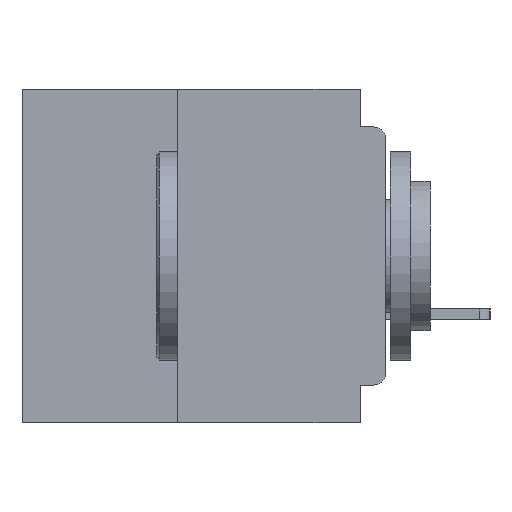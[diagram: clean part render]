
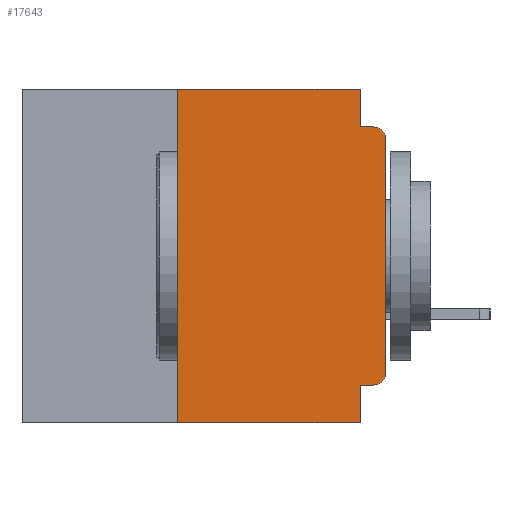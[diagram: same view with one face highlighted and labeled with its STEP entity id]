
A CAD part, left-side view. The second image highlights one B-rep face of the part: STEP entity #17643.
In plain terms, the highlighted planar face has unit normal (-1, 0, 0).
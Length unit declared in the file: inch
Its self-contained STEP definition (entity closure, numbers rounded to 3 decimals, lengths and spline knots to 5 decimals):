
#552 = DIRECTION ( 'NONE',  ( -1., 0., 0. ) ) ;
#1470 = LINE ( 'NONE', #4682, #11370 ) ;
#1479 = CARTESIAN_POINT ( 'NONE',  ( 0., 0.031, -0.4 ) ) ;
#1695 = DIRECTION ( 'NONE',  ( 0., 1., 0. ) ) ;
#1848 = VERTEX_POINT ( 'NONE', #18708 ) ;
#2295 = EDGE_CURVE ( 'NONE', #50090, #1848, #46483, .T. ) ;
#2937 = EDGE_CURVE ( 'NONE', #40375, #10852, #7028, .T. ) ;
#3346 = EDGE_CURVE ( 'NONE', #35002, #20147, #49579, .T. ) ;
#4307 = CARTESIAN_POINT ( 'NONE',  ( 0., 0., 0. ) ) ;
#4682 = CARTESIAN_POINT ( 'NONE',  ( 0., 0.031, 0. ) ) ;
#5439 = ORIENTED_EDGE ( 'NONE', *, *, #36839, .F. ) ;
#5777 = EDGE_CURVE ( 'NONE', #19562, #10852, #32001, .T. ) ;
#6863 = VERTEX_POINT ( 'NONE', #14213 ) ;
#7028 = LINE ( 'NONE', #52720, #16855 ) ;
#8505 = AXIS2_PLACEMENT_3D ( 'NONE', #49278, #53401, #28802 ) ;
#8623 = EDGE_CURVE ( 'NONE', #19562, #12308, #39413, .T. ) ;
#8981 = CIRCLE ( 'NONE', #23142, 0.015 ) ;
#8997 = ORIENTED_EDGE ( 'NONE', *, *, #5777, .T. ) ;
#9001 = EDGE_CURVE ( 'NONE', #17602, #1848, #8981, .T. ) ;
#10029 = VECTOR ( 'NONE', #27880, 39.37008 ) ;
#10455 = ORIENTED_EDGE ( 'NONE', *, *, #3346, .T. ) ;
#10621 = LINE ( 'NONE', #43025, #42249 ) ;
#10852 = VERTEX_POINT ( 'NONE', #1479 ) ;
#11066 = ORIENTED_EDGE ( 'NONE', *, *, #38443, .T. ) ;
#11228 = CARTESIAN_POINT ( 'NONE',  ( 0., 0.437, -0.4 ) ) ;
#11370 = VECTOR ( 'NONE', #25450, 39.37008 ) ;
#12308 = VERTEX_POINT ( 'NONE', #48574 ) ;
#12847 = CARTESIAN_POINT ( 'NONE',  ( 0., 0.015, -0.355 ) ) ;
#14213 = CARTESIAN_POINT ( 'NONE',  ( 0., 0.031, 0. ) ) ;
#14452 = CARTESIAN_POINT ( 'NONE',  ( 0., 0.25, -0.4 ) ) ;
#14571 = ORIENTED_EDGE ( 'NONE', *, *, #9001, .T. ) ;
#15018 = AXIS2_PLACEMENT_3D ( 'NONE', #42183, #42110, #41984 ) ;
#16855 = VECTOR ( 'NONE', #52776, 39.37008 ) ;
#17497 = EDGE_LOOP ( 'NONE', ( #11066, #14571, #36678, #48957, #5439, #48755, #8997, #39655, #50337, #10455 ) ) ;
#17602 = VERTEX_POINT ( 'NONE', #32575 ) ;
#17643 = ADVANCED_FACE ( 'NONE', ( #43228 ), #20543, .F. ) ;
#18305 = LINE ( 'NONE', #50562, #40161 ) ;
#18708 = CARTESIAN_POINT ( 'NONE',  ( 0., 0.015, -0.045 ) ) ;
#18836 = VECTOR ( 'NONE', #48781, 39.37008 ) ;
#19562 = VERTEX_POINT ( 'NONE', #28008 ) ;
#19796 = EDGE_CURVE ( 'NONE', #6863, #50090, #1470, .T. ) ;
#20147 = VERTEX_POINT ( 'NONE', #32768 ) ;
#20543 = PLANE ( 'NONE',  #8505 ) ;
#21846 = DIRECTION ( 'NONE',  ( 0., -1., 0. ) ) ;
#23142 = AXIS2_PLACEMENT_3D ( 'NONE', #25586, #552, #29713 ) ;
#23813 = CARTESIAN_POINT ( 'NONE',  ( 0., 0.031, -0.045 ) ) ;
#24668 = VECTOR ( 'NONE', #41869, 39.37008 ) ;
#25450 = DIRECTION ( 'NONE',  ( 0., 0., -1. ) ) ;
#25586 = CARTESIAN_POINT ( 'NONE',  ( 0., 0.015, -0.06 ) ) ;
#25716 = EDGE_CURVE ( 'NONE', #35002, #40375, #10621, .T. ) ;
#26926 = DIRECTION ( 'NONE',  ( 0., 0., 1. ) ) ;
#27880 = DIRECTION ( 'NONE',  ( 0., -1., 0. ) ) ;
#28008 = CARTESIAN_POINT ( 'NONE',  ( 0., 0.25, -0.4 ) ) ;
#28483 = VECTOR ( 'NONE', #26926, 39.37008 ) ;
#28802 = DIRECTION ( 'NONE',  ( 0., 0., -1. ) ) ;
#29713 = DIRECTION ( 'NONE',  ( 0., 0., -1. ) ) ;
#32001 = LINE ( 'NONE', #11228, #10029 ) ;
#32575 = CARTESIAN_POINT ( 'NONE',  ( 0., 0., -0.06 ) ) ;
#32768 = CARTESIAN_POINT ( 'NONE',  ( 0., 0., -0.34 ) ) ;
#35002 = VERTEX_POINT ( 'NONE', #12847 ) ;
#36678 = ORIENTED_EDGE ( 'NONE', *, *, #2295, .F. ) ;
#36839 = EDGE_CURVE ( 'NONE', #12308, #6863, #18305, .T. ) ;
#38443 = EDGE_CURVE ( 'NONE', #20147, #17602, #51621, .T. ) ;
#39413 = LINE ( 'NONE', #14452, #28483 ) ;
#39655 = ORIENTED_EDGE ( 'NONE', *, *, #2937, .F. ) ;
#40161 = VECTOR ( 'NONE', #21846, 39.37008 ) ;
#40375 = VERTEX_POINT ( 'NONE', #50214 ) ;
#41869 = DIRECTION ( 'NONE',  ( 0., -1., 0. ) ) ;
#41984 = DIRECTION ( 'NONE',  ( 0., 0., -1. ) ) ;
#42055 = CARTESIAN_POINT ( 'NONE',  ( 0., 0., -0.045 ) ) ;
#42110 = DIRECTION ( 'NONE',  ( -1., 0., 0. ) ) ;
#42183 = CARTESIAN_POINT ( 'NONE',  ( 0., 0.015, -0.34 ) ) ;
#42249 = VECTOR ( 'NONE', #1695, 39.37008 ) ;
#43025 = CARTESIAN_POINT ( 'NONE',  ( 0., 0., -0.355 ) ) ;
#43228 = FACE_OUTER_BOUND ( 'NONE', #17497, .T. ) ;
#46483 = LINE ( 'NONE', #42055, #24668 ) ;
#48574 = CARTESIAN_POINT ( 'NONE',  ( 0., 0.25, 0. ) ) ;
#48755 = ORIENTED_EDGE ( 'NONE', *, *, #8623, .F. ) ;
#48781 = DIRECTION ( 'NONE',  ( 0., 0., 1. ) ) ;
#48957 = ORIENTED_EDGE ( 'NONE', *, *, #19796, .F. ) ;
#49278 = CARTESIAN_POINT ( 'NONE',  ( 0., 0.437, 0. ) ) ;
#49579 = CIRCLE ( 'NONE', #15018, 0.015 ) ;
#50090 = VERTEX_POINT ( 'NONE', #23813 ) ;
#50214 = CARTESIAN_POINT ( 'NONE',  ( 0., 0.031, -0.355 ) ) ;
#50337 = ORIENTED_EDGE ( 'NONE', *, *, #25716, .F. ) ;
#50562 = CARTESIAN_POINT ( 'NONE',  ( 0., 0.437, 0. ) ) ;
#51621 = LINE ( 'NONE', #4307, #18836 ) ;
#52720 = CARTESIAN_POINT ( 'NONE',  ( 0., 0.031, -0.4 ) ) ;
#52776 = DIRECTION ( 'NONE',  ( 0., 0., -1. ) ) ;
#53401 = DIRECTION ( 'NONE',  ( 1., 0., 0. ) ) ;
